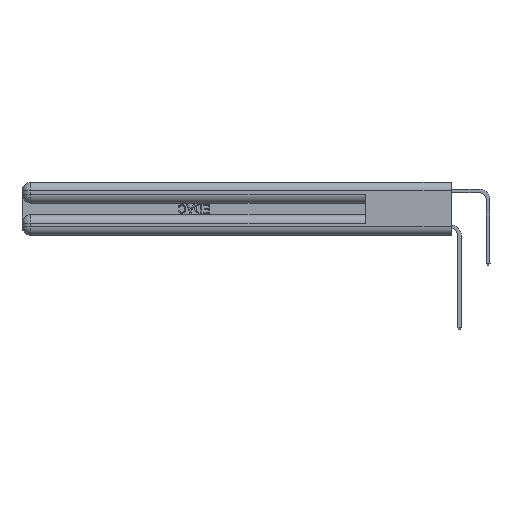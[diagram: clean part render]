
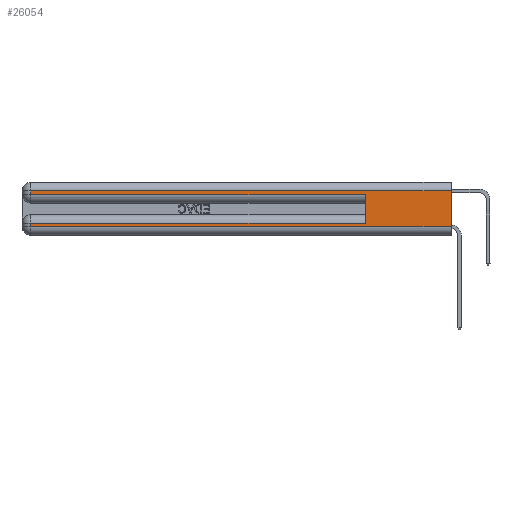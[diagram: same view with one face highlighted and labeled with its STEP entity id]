
A CAD part, left-side view. The second image highlights one B-rep face of the part: STEP entity #26054.
In plain terms, the highlighted planar face has unit normal (-1, 0, 0).
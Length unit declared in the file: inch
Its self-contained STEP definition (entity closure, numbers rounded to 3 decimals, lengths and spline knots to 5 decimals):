
#520 = EDGE_CURVE ( 'NONE', #9659, #6777, #22344, .T. ) ;
#906 = CARTESIAN_POINT ( 'NONE',  ( 0., 0., 0.37 ) ) ;
#1104 = LINE ( 'NONE', #23986, #8697 ) ;
#1407 = PLANE ( 'NONE',  #30654 ) ;
#2074 = EDGE_CURVE ( 'NONE', #18844, #21156, #17425, .T. ) ;
#2587 = EDGE_CURVE ( 'NONE', #23007, #9659, #22806, .T. ) ;
#3405 = ORIENTED_EDGE ( 'NONE', *, *, #20679, .T. ) ;
#4064 = CARTESIAN_POINT ( 'NONE',  ( 0., 0., 0.06 ) ) ;
#4654 = CARTESIAN_POINT ( 'NONE',  ( 0., 0.6, 0.085 ) ) ;
#4684 = VECTOR ( 'NONE', #16009, 39.37008 ) ;
#5552 = EDGE_LOOP ( 'NONE', ( #24896, #27257, #16271, #3405, #16530, #7992, #21522, #22288 ) ) ;
#5668 = LINE ( 'NONE', #15805, #10899 ) ;
#6777 = VERTEX_POINT ( 'NONE', #11949 ) ;
#7992 = ORIENTED_EDGE ( 'NONE', *, *, #2587, .T. ) ;
#8460 = LINE ( 'NONE', #8620, #31449 ) ;
#8620 = CARTESIAN_POINT ( 'NONE',  ( 0., 0., 0.31 ) ) ;
#8697 = VECTOR ( 'NONE', #18866, 39.37008 ) ;
#8990 = DIRECTION ( 'NONE',  ( 0., -1., 0. ) ) ;
#9659 = VERTEX_POINT ( 'NONE', #21126 ) ;
#10028 = DIRECTION ( 'NONE',  ( 0., 1., 0. ) ) ;
#10833 = VECTOR ( 'NONE', #15082, 39.37008 ) ;
#10899 = VECTOR ( 'NONE', #8990, 39.37008 ) ;
#11018 = FACE_OUTER_BOUND ( 'NONE', #5552, .T. ) ;
#11436 = EDGE_CURVE ( 'NONE', #18844, #14783, #8460, .T. ) ;
#11521 = DIRECTION ( 'NONE',  ( 0., 0., -1. ) ) ;
#11949 = CARTESIAN_POINT ( 'NONE',  ( 0., 2.94, 0.06 ) ) ;
#13322 = CARTESIAN_POINT ( 'NONE',  ( 0., 0., 0.06 ) ) ;
#13648 = EDGE_CURVE ( 'NONE', #6777, #21156, #18519, .T. ) ;
#14783 = VERTEX_POINT ( 'NONE', #28017 ) ;
#15082 = DIRECTION ( 'NONE',  ( 0., 0., -1. ) ) ;
#15805 = CARTESIAN_POINT ( 'NONE',  ( 0., 0., 0.285 ) ) ;
#16009 = DIRECTION ( 'NONE',  ( 0., -1., 0. ) ) ;
#16091 = EDGE_CURVE ( 'NONE', #14783, #17931, #25697, .T. ) ;
#16271 = ORIENTED_EDGE ( 'NONE', *, *, #16091, .T. ) ;
#16530 = ORIENTED_EDGE ( 'NONE', *, *, #17487, .F. ) ;
#17425 = LINE ( 'NONE', #24724, #26176 ) ;
#17487 = EDGE_CURVE ( 'NONE', #23007, #18963, #1104, .T. ) ;
#17931 = VERTEX_POINT ( 'NONE', #29219 ) ;
#18519 = LINE ( 'NONE', #4064, #4684 ) ;
#18844 = VERTEX_POINT ( 'NONE', #29303 ) ;
#18866 = DIRECTION ( 'NONE',  ( 0., 0., 1. ) ) ;
#18963 = VERTEX_POINT ( 'NONE', #30126 ) ;
#20679 = EDGE_CURVE ( 'NONE', #17931, #18963, #5668, .T. ) ;
#21126 = CARTESIAN_POINT ( 'NONE',  ( 0., 2.94, 0.085 ) ) ;
#21156 = VERTEX_POINT ( 'NONE', #13322 ) ;
#21522 = ORIENTED_EDGE ( 'NONE', *, *, #520, .T. ) ;
#22288 = ORIENTED_EDGE ( 'NONE', *, *, #13648, .T. ) ;
#22344 = LINE ( 'NONE', #32442, #32430 ) ;
#22806 = LINE ( 'NONE', #24361, #29894 ) ;
#23007 = VERTEX_POINT ( 'NONE', #4654 ) ;
#23986 = CARTESIAN_POINT ( 'NONE',  ( 0., 0.6, 0.145 ) ) ;
#24361 = CARTESIAN_POINT ( 'NONE',  ( 0., 0., 0.085 ) ) ;
#24400 = DIRECTION ( 'NONE',  ( 0., 0., -1. ) ) ;
#24724 = CARTESIAN_POINT ( 'NONE',  ( 0., 0., 0.37 ) ) ;
#24896 = ORIENTED_EDGE ( 'NONE', *, *, #2074, .F. ) ;
#25697 = LINE ( 'NONE', #27862, #10833 ) ;
#26054 = ADVANCED_FACE ( 'NONE', ( #11018 ), #1407, .F. ) ;
#26176 = VECTOR ( 'NONE', #24400, 39.37008 ) ;
#26786 = DIRECTION ( 'NONE',  ( 1., 0., 0. ) ) ;
#27257 = ORIENTED_EDGE ( 'NONE', *, *, #11436, .T. ) ;
#27862 = CARTESIAN_POINT ( 'NONE',  ( 0., 2.94, 0.37 ) ) ;
#28017 = CARTESIAN_POINT ( 'NONE',  ( 0., 2.94, 0.31 ) ) ;
#28877 = DIRECTION ( 'NONE',  ( 0., 1., 0. ) ) ;
#29219 = CARTESIAN_POINT ( 'NONE',  ( 0., 2.94, 0.285 ) ) ;
#29303 = CARTESIAN_POINT ( 'NONE',  ( 0., 0., 0.31 ) ) ;
#29894 = VECTOR ( 'NONE', #10028, 39.37008 ) ;
#30126 = CARTESIAN_POINT ( 'NONE',  ( 0., 0.6, 0.285 ) ) ;
#30132 = DIRECTION ( 'NONE',  ( 0., 0., -1. ) ) ;
#30654 = AXIS2_PLACEMENT_3D ( 'NONE', #906, #26786, #11521 ) ;
#31449 = VECTOR ( 'NONE', #28877, 39.37008 ) ;
#32430 = VECTOR ( 'NONE', #30132, 39.37008 ) ;
#32442 = CARTESIAN_POINT ( 'NONE',  ( 0., 2.94, 0.37 ) ) ;
